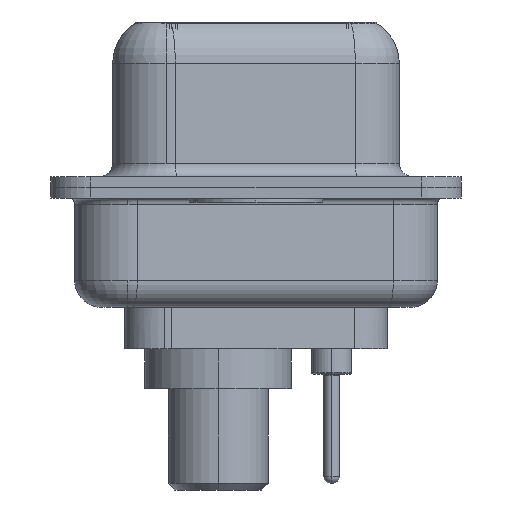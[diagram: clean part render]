
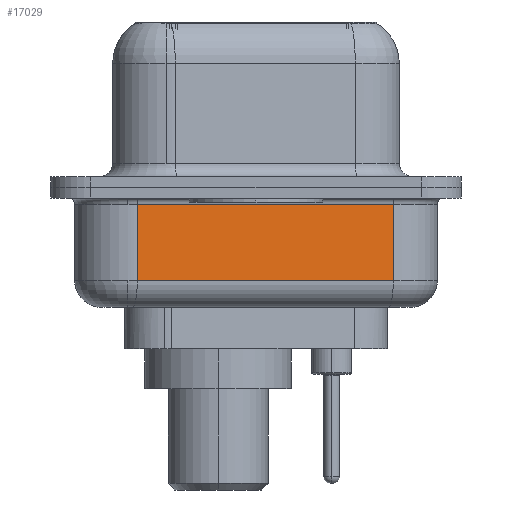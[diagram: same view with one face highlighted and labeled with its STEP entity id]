
A CAD part, left-side view. The second image highlights one B-rep face of the part: STEP entity #17029.
In plain terms, the highlighted planar face has unit normal (-0.985, -0.174, 0).
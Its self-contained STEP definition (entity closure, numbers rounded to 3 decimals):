
#290 = DIRECTION ( 'NONE',  ( -0.174, 0.985, 0. ) ) ;
#546 = CARTESIAN_POINT ( 'NONE',  ( 2.93, 4.453, -0.65 ) ) ;
#1328 = VECTOR ( 'NONE', #9969, 1000. ) ;
#1601 = ORIENTED_EDGE ( 'NONE', *, *, #10011, .T. ) ;
#1853 = ORIENTED_EDGE ( 'NONE', *, *, #22595, .F. ) ;
#2177 = ORIENTED_EDGE ( 'NONE', *, *, #10780, .T. ) ;
#2837 = ORIENTED_EDGE ( 'NONE', *, *, #28677, .T. ) ;
#3584 = DIRECTION ( 'NONE',  ( 0., 0., 1. ) ) ;
#3701 = DIRECTION ( 'NONE',  ( 0.174, -0.985, 0. ) ) ;
#4031 = CARTESIAN_POINT ( 'NONE',  ( 2.93, 4.453, -3.5 ) ) ;
#6219 = CARTESIAN_POINT ( 'NONE',  ( 2.93, 4.453, -3.5 ) ) ;
#6261 = CARTESIAN_POINT ( 'NONE',  ( 4.623, -5.147, -3.5 ) ) ;
#9566 = VERTEX_POINT ( 'NONE', #6261 ) ;
#9805 = LINE ( 'NONE', #13171, #20070 ) ;
#9969 = DIRECTION ( 'NONE',  ( -0.174, 0.985, 0. ) ) ;
#10011 = EDGE_CURVE ( 'NONE', #19555, #9566, #29944, .T. ) ;
#10780 = EDGE_CURVE ( 'NONE', #11703, #12423, #14844, .T. ) ;
#11703 = VERTEX_POINT ( 'NONE', #27859 ) ;
#12423 = VERTEX_POINT ( 'NONE', #546 ) ;
#13171 = CARTESIAN_POINT ( 'NONE',  ( 4.623, -5.147, -4.5 ) ) ;
#14300 = DIRECTION ( 'NONE',  ( 0.985, 0.174, 0. ) ) ;
#14844 = LINE ( 'NONE', #26272, #1328 ) ;
#15176 = EDGE_LOOP ( 'NONE', ( #1853, #1601, #2837, #2177 ) ) ;
#15608 = VECTOR ( 'NONE', #3701, 1000. ) ;
#16080 = FACE_OUTER_BOUND ( 'NONE', #15176, .T. ) ;
#17029 = ADVANCED_FACE ( 'NONE', ( #16080 ), #23639, .F. ) ;
#19555 = VERTEX_POINT ( 'NONE', #4031 ) ;
#20070 = VECTOR ( 'NONE', #3584, 1000. ) ;
#20440 = AXIS2_PLACEMENT_3D ( 'NONE', #28383, #14300, #290 ) ;
#22460 = CARTESIAN_POINT ( 'NONE',  ( 2.93, 4.453, -4.5 ) ) ;
#22595 = EDGE_CURVE ( 'NONE', #19555, #12423, #27612, .T. ) ;
#23639 = PLANE ( 'NONE',  #20440 ) ;
#25614 = DIRECTION ( 'NONE',  ( 0., 0., 1. ) ) ;
#26272 = CARTESIAN_POINT ( 'NONE',  ( 2.93, 4.453, -0.65 ) ) ;
#27612 = LINE ( 'NONE', #22460, #27986 ) ;
#27859 = CARTESIAN_POINT ( 'NONE',  ( 4.623, -5.147, -0.65 ) ) ;
#27986 = VECTOR ( 'NONE', #25614, 1000. ) ;
#28383 = CARTESIAN_POINT ( 'NONE',  ( 2.93, 4.453, -4.5 ) ) ;
#28677 = EDGE_CURVE ( 'NONE', #9566, #11703, #9805, .T. ) ;
#29944 = LINE ( 'NONE', #6219, #15608 ) ;
